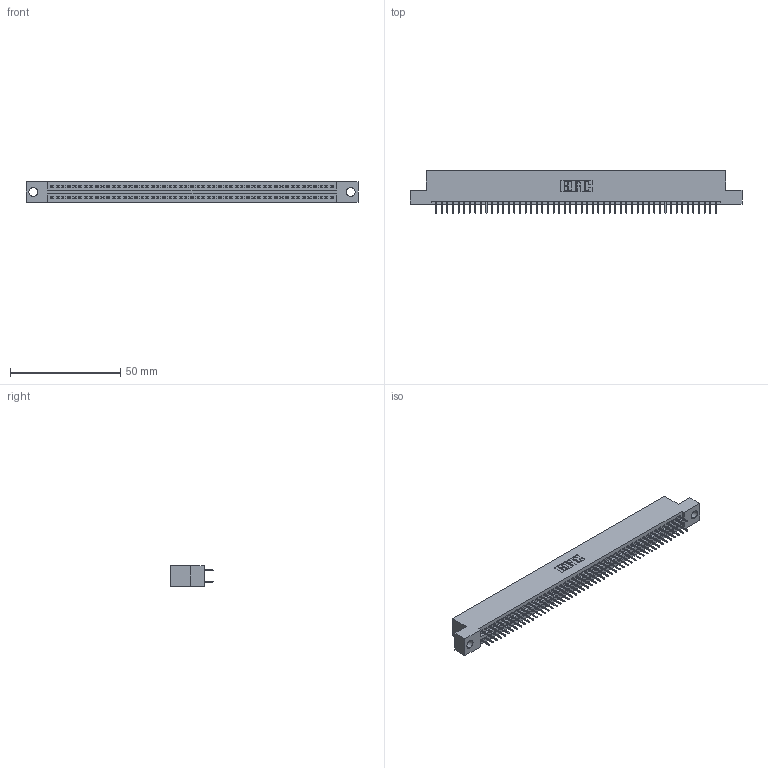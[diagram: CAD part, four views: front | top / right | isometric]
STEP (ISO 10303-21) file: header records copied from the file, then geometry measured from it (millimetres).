
FILE_DESCRIPTION (( 'STEP AP203' ), '1' );
FILE_NAME ('395-102-524-204.STEP', '2018-11-30T06:19:40', ( '' ), ( '' ), 'SwSTEP 2.0', 'SolidWorks 2016', '' );
FILE_SCHEMA (( 'CONFIG_CONTROL_DESIGN' ));
Length unit declared in the file: inch
Products named in the file (3): 395-102-524-204; 345 Part_Flush Mounting Lugs - 0.156 Dia-TH; 345-292-001_345-293-124
Assembly tree (103 placements, depth 2):
  395-102-524-204
    345 Part_Flush Mounting Lugs - 0.156 Dia-TH
    345-292-001_345-293-124  x102
Bounding box: 150.75 x 19.35 x 9.4 mm (x, y, z)
Volume: 14485.2 mm3; surface area: 20993.6 mm2
Topology: 103 solids, 103 shells, 5634 faces, 15947 edges, 10222 vertices
Faces by surface type: plane 4058, cylinder 1576
Entity records: 38881 total; most frequent: CARTESIAN_POINT 6508, ORIENTED_EDGE 6442, DIRECTION 5729, EDGE_CURVE 3221, LINE 2889, VECTOR 2889, VERTEX_POINT 2142, AXIS2_PLACEMENT_3D 1420
